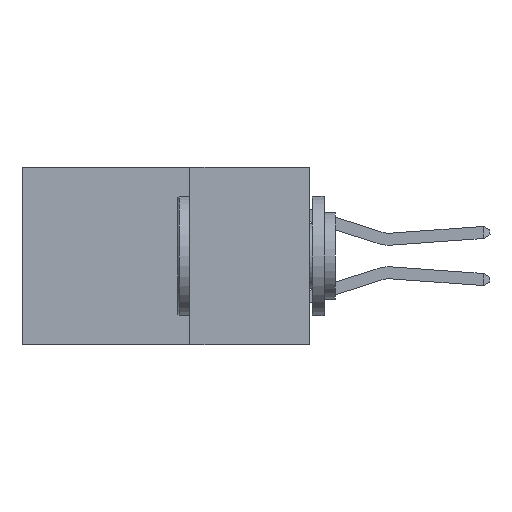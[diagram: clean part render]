
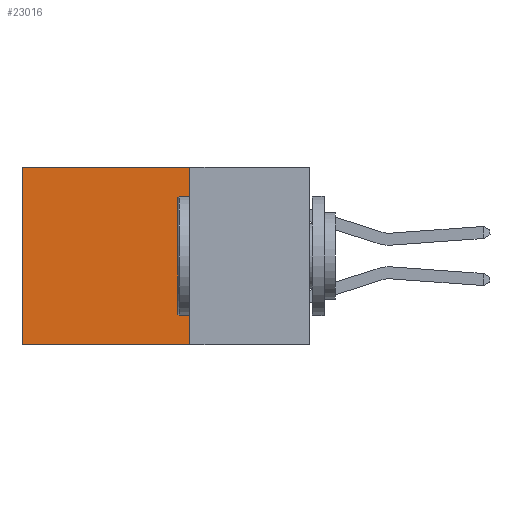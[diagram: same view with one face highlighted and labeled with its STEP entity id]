
A CAD part, left-side view. The second image highlights one B-rep face of the part: STEP entity #23016.
In plain terms, the highlighted planar face has unit normal (-1, 0, 0).
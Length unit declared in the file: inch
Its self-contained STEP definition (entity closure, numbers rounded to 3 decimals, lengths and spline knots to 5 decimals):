
#673 = VECTOR ( 'NONE', #21563, 39.37008 ) ;
#718 = LINE ( 'NONE', #13517, #20702 ) ;
#806 = CARTESIAN_POINT ( 'NONE',  ( 0.298, 0.25, 0. ) ) ;
#836 = ORIENTED_EDGE ( 'NONE', *, *, #16532, .T. ) ;
#2180 = FACE_OUTER_BOUND ( 'NONE', #11980, .T. ) ;
#2223 = ORIENTED_EDGE ( 'NONE', *, *, #4791, .F. ) ;
#2428 = DIRECTION ( 'NONE',  ( 0., 1., 0. ) ) ;
#2634 = DIRECTION ( 'NONE',  ( 1., 0., 0. ) ) ;
#4630 = CARTESIAN_POINT ( 'NONE',  ( 0.298, 0.25, 0. ) ) ;
#4791 = EDGE_CURVE ( 'NONE', #13918, #14825, #21812, .T. ) ;
#6168 = DIRECTION ( 'NONE',  ( 0., 0., -1. ) ) ;
#7607 = CARTESIAN_POINT ( 'NONE',  ( 0.298, 0.25, -0.37 ) ) ;
#8007 = DIRECTION ( 'NONE',  ( 0., 1., 0. ) ) ;
#9243 = EDGE_CURVE ( 'NONE', #13815, #14825, #14652, .T. ) ;
#10846 = LINE ( 'NONE', #20552, #15173 ) ;
#10926 = CARTESIAN_POINT ( 'NONE',  ( 0.298, 0.6, 0. ) ) ;
#11769 = VERTEX_POINT ( 'NONE', #4630 ) ;
#11980 = EDGE_LOOP ( 'NONE', ( #14628, #2223, #18924, #836 ) ) ;
#13051 = CARTESIAN_POINT ( 'NONE',  ( 0.298, 0.6, -0.37 ) ) ;
#13517 = CARTESIAN_POINT ( 'NONE',  ( 0.298, 0.25, 0. ) ) ;
#13815 = VERTEX_POINT ( 'NONE', #18423 ) ;
#13918 = VERTEX_POINT ( 'NONE', #18052 ) ;
#14628 = ORIENTED_EDGE ( 'NONE', *, *, #9243, .T. ) ;
#14652 = LINE ( 'NONE', #10926, #673 ) ;
#14825 = VERTEX_POINT ( 'NONE', #13051 ) ;
#15173 = VECTOR ( 'NONE', #6168, 39.37008 ) ;
#16532 = EDGE_CURVE ( 'NONE', #11769, #13815, #718, .T. ) ;
#18052 = CARTESIAN_POINT ( 'NONE',  ( 0.298, 0.25, -0.37 ) ) ;
#18270 = EDGE_CURVE ( 'NONE', #11769, #13918, #10846, .T. ) ;
#18423 = CARTESIAN_POINT ( 'NONE',  ( 0.298, 0.6, 0. ) ) ;
#18685 = VECTOR ( 'NONE', #2428, 39.37008 ) ;
#18924 = ORIENTED_EDGE ( 'NONE', *, *, #18270, .F. ) ;
#19073 = DIRECTION ( 'NONE',  ( 0., 0., -1. ) ) ;
#20552 = CARTESIAN_POINT ( 'NONE',  ( 0.298, 0.25, 0. ) ) ;
#20702 = VECTOR ( 'NONE', #8007, 39.37008 ) ;
#21563 = DIRECTION ( 'NONE',  ( 0., 0., -1. ) ) ;
#21812 = LINE ( 'NONE', #7607, #18685 ) ;
#22028 = AXIS2_PLACEMENT_3D ( 'NONE', #806, #2634, #19073 ) ;
#22125 = PLANE ( 'NONE',  #22028 ) ;
#23016 = ADVANCED_FACE ( 'NONE', ( #2180 ), #22125, .F. ) ;
